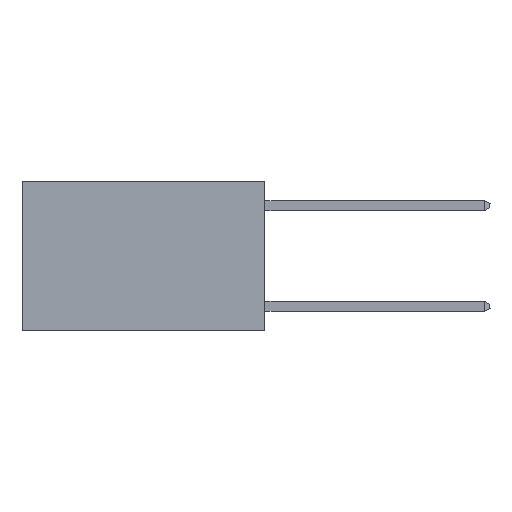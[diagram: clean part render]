
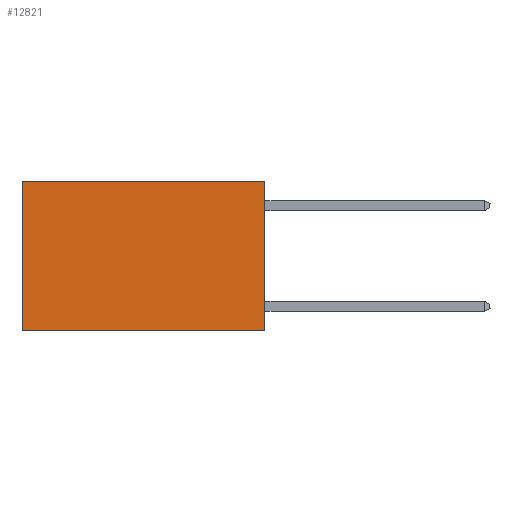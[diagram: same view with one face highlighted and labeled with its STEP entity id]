
A CAD part, left-side view. The second image highlights one B-rep face of the part: STEP entity #12821.
In plain terms, the highlighted planar face has unit normal (-1, 0, 0).
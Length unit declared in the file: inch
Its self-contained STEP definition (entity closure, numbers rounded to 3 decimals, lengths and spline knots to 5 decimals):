
#726 = VERTEX_POINT ( 'NONE', #19467 ) ;
#1598 = VERTEX_POINT ( 'NONE', #3828 ) ;
#3448 = VECTOR ( 'NONE', #21798, 39.37008 ) ;
#3828 = CARTESIAN_POINT ( 'NONE',  ( 0.2625, 0., -0.37 ) ) ;
#4316 = CARTESIAN_POINT ( 'NONE',  ( 0.2625, 0., 0. ) ) ;
#5292 = CARTESIAN_POINT ( 'NONE',  ( 0.2625, 0., 0. ) ) ;
#5766 = AXIS2_PLACEMENT_3D ( 'NONE', #15894, #16135, #23382 ) ;
#5831 = EDGE_CURVE ( 'NONE', #726, #15658, #12954, .T. ) ;
#6250 = CARTESIAN_POINT ( 'NONE',  ( 0.2625, 0., 0. ) ) ;
#6487 = VECTOR ( 'NONE', #10702, 39.37008 ) ;
#8545 = PLANE ( 'NONE',  #5766 ) ;
#9296 = VECTOR ( 'NONE', #15024, 39.37008 ) ;
#9471 = EDGE_CURVE ( 'NONE', #18738, #726, #14210, .T. ) ;
#10475 = DIRECTION ( 'NONE',  ( 0., 1., 0. ) ) ;
#10702 = DIRECTION ( 'NONE',  ( 0., 0., -1. ) ) ;
#10718 = CARTESIAN_POINT ( 'NONE',  ( 0.2625, 0., -0.37 ) ) ;
#10848 = LINE ( 'NONE', #10718, #19961 ) ;
#11121 = CARTESIAN_POINT ( 'NONE',  ( 0.2625, 0.6, -0.37 ) ) ;
#12607 = ORIENTED_EDGE ( 'NONE', *, *, #5831, .T. ) ;
#12742 = ORIENTED_EDGE ( 'NONE', *, *, #9471, .T. ) ;
#12821 = ADVANCED_FACE ( 'NONE', ( #17648 ), #8545, .F. ) ;
#12954 = LINE ( 'NONE', #14693, #6487 ) ;
#14210 = LINE ( 'NONE', #6250, #3448 ) ;
#14693 = CARTESIAN_POINT ( 'NONE',  ( 0.2625, 0.6, 0. ) ) ;
#15024 = DIRECTION ( 'NONE',  ( 0., 0., -1. ) ) ;
#15658 = VERTEX_POINT ( 'NONE', #11121 ) ;
#15894 = CARTESIAN_POINT ( 'NONE',  ( 0.2625, 0., 0. ) ) ;
#16135 = DIRECTION ( 'NONE',  ( 1., 0., 0. ) ) ;
#16354 = EDGE_LOOP ( 'NONE', ( #12607, #17362, #19724, #12742 ) ) ;
#17362 = ORIENTED_EDGE ( 'NONE', *, *, #19249, .F. ) ;
#17648 = FACE_OUTER_BOUND ( 'NONE', #16354, .T. ) ;
#18738 = VERTEX_POINT ( 'NONE', #4316 ) ;
#19249 = EDGE_CURVE ( 'NONE', #1598, #15658, #10848, .T. ) ;
#19467 = CARTESIAN_POINT ( 'NONE',  ( 0.2625, 0.6, 0. ) ) ;
#19724 = ORIENTED_EDGE ( 'NONE', *, *, #23735, .F. ) ;
#19961 = VECTOR ( 'NONE', #10475, 39.37008 ) ;
#21798 = DIRECTION ( 'NONE',  ( 0., 1., 0. ) ) ;
#23382 = DIRECTION ( 'NONE',  ( 0., 0., -1. ) ) ;
#23735 = EDGE_CURVE ( 'NONE', #18738, #1598, #24376, .T. ) ;
#24376 = LINE ( 'NONE', #5292, #9296 ) ;
